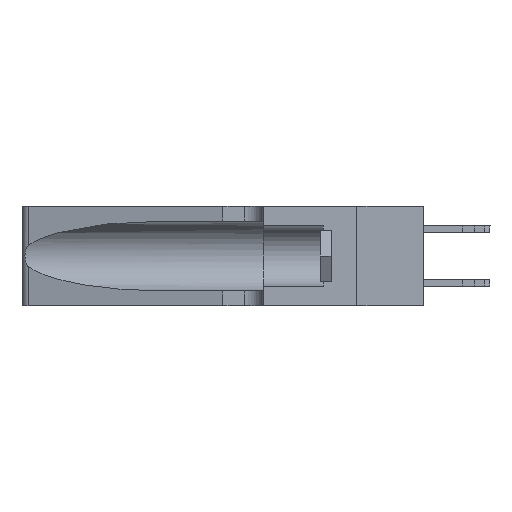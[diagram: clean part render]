
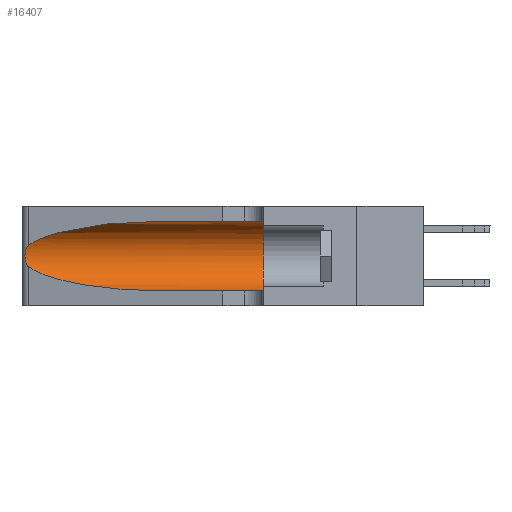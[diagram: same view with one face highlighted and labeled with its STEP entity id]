
A CAD part, left-side view. The second image highlights one B-rep face of the part: STEP entity #16407.
In plain terms, the highlighted cylindrical face has radius 3.308 mm (diameter 6.617 mm), a partial arc.
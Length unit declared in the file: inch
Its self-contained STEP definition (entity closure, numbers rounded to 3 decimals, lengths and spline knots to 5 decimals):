
#221 = CIRCLE ( 'NONE', #20398, 0.13025 ) ;
#550 = CARTESIAN_POINT ( 'NONE',  ( 0.1305, 0.72297, 0.31525 ) ) ;
#918 = VERTEX_POINT ( 'NONE', #16418 ) ;
#952 = EDGE_CURVE ( 'NONE', #918, #15052, #13088, .T. ) ;
#955 = ORIENTED_EDGE ( 'NONE', *, *, #3729, .F. ) ;
#1176 = CYLINDRICAL_SURFACE ( 'NONE', #19075, 0.13025 ) ;
#1247 = CARTESIAN_POINT ( 'NONE',  ( 0.25639, 1.23186, 0.15144 ) ) ;
#1499 = ORIENTED_EDGE ( 'NONE', *, *, #3423, .T. ) ;
#3002 = CARTESIAN_POINT ( 'NONE',  ( 0.26075, 1.23896, 0.178 ) ) ;
#3423 = EDGE_CURVE ( 'NONE', #6405, #12918, #13375, .T. ) ;
#3729 = EDGE_CURVE ( 'NONE', #11415, #15052, #221, .T. ) ;
#3819 = CARTESIAN_POINT ( 'NONE',  ( 0.2373, 1.15595, 0.28018 ) ) ;
#4399 = EDGE_CURVE ( 'NONE', #7703, #11415, #8384, .T. ) ;
#4429 = CARTESIAN_POINT ( 'NONE',  ( 0.25555, 1.22993, 0.14849 ) ) ;
#5075 = DIRECTION ( 'NONE',  ( 0., 0., -1. ) ) ;
#5681 = CARTESIAN_POINT ( 'NONE',  ( 0.25487, 1.22718, 0.14631 ) ) ;
#6241 = CARTESIAN_POINT ( 'NONE',  ( 0.25639, 1.23184, 0.21858 ) ) ;
#6405 = VERTEX_POINT ( 'NONE', #19972 ) ;
#6796 = CARTESIAN_POINT ( 'NONE',  ( 0.18966, 0.96281, 0.31525 ) ) ;
#6901 = CARTESIAN_POINT ( 'NONE',  ( 0.1305, 0.35, 0.31525 ) ) ;
#7072 = ORIENTED_EDGE ( 'NONE', *, *, #15468, .T. ) ;
#7164 =( BOUNDED_CURVE ( )  B_SPLINE_CURVE ( 3, ( #14994, #16622, #8827, #18570 ),
 .UNSPECIFIED., .F., .F. ) 
 B_SPLINE_CURVE_WITH_KNOTS ( ( 4, 4 ),
 ( 3.44316, 4.71239 ),
 .UNSPECIFIED. ) 
 CURVE ( )  GEOMETRIC_REPRESENTATION_ITEM ( )  RATIONAL_B_SPLINE_CURVE ( ( 1., 0.87, 0.87, 1. ) ) 
 REPRESENTATION_ITEM ( '' )  );
#7393 = FACE_OUTER_BOUND ( 'NONE', #14628, .T. ) ;
#7504 = CARTESIAN_POINT ( 'NONE',  ( 0.1305, 1.61858, 0.05475 ) ) ;
#7569 = DIRECTION ( 'NONE',  ( 0., -1., 0. ) ) ;
#7703 = VERTEX_POINT ( 'NONE', #550 ) ;
#7839 = CARTESIAN_POINT ( 'NONE',  ( 0.25854, 1.2359, 0.20912 ) ) ;
#8062 =( BOUNDED_CURVE ( )  B_SPLINE_CURVE ( 3, ( #13434, #6796, #3819, #16614 ),
 .UNSPECIFIED., .F., .T. ) 
 B_SPLINE_CURVE_WITH_KNOTS ( ( 4, 4 ),
 ( 1.5708, 2.84003 ),
 .UNSPECIFIED. ) 
 CURVE ( )  GEOMETRIC_REPRESENTATION_ITEM ( )  RATIONAL_B_SPLINE_CURVE ( ( 1., 0.87, 0.87, 1. ) ) 
 REPRESENTATION_ITEM ( '' )  );
#8350 = DIRECTION ( 'NONE',  ( 0., 1., 0. ) ) ;
#8384 = LINE ( 'NONE', #19009, #18735 ) ;
#8827 = CARTESIAN_POINT ( 'NONE',  ( 0.18966, 0.96281, 0.05475 ) ) ;
#9008 = EDGE_CURVE ( 'NONE', #7703, #6405, #8062, .T. ) ;
#9167 = CARTESIAN_POINT ( 'NONE',  ( 0.25555, 1.22994, 0.2215 ) ) ;
#9451 = CARTESIAN_POINT ( 'NONE',  ( 0.26017, 1.23833, 0.17102 ) ) ;
#9759 = CARTESIAN_POINT ( 'NONE',  ( 0.1305, 1.61858, 0.185 ) ) ;
#9830 = CARTESIAN_POINT ( 'NONE',  ( 0.1305, 0.35, 0.05475 ) ) ;
#10783 = CARTESIAN_POINT ( 'NONE',  ( 0.26018, 1.23835, 0.19895 ) ) ;
#11379 = DIRECTION ( 'NONE',  ( 0., -1., 0. ) ) ;
#11415 = VERTEX_POINT ( 'NONE', #6901 ) ;
#11594 = DIRECTION ( 'NONE',  ( 0., 0., 1. ) ) ;
#12589 = VECTOR ( 'NONE', #7569, 39.37008 ) ;
#12918 = VERTEX_POINT ( 'NONE', #5681 ) ;
#13088 = LINE ( 'NONE', #7504, #12589 ) ;
#13375 = B_SPLINE_CURVE_WITH_KNOTS ( 'NONE', 3,
 ( #15909, #9167, #6241, #17499, #7839, #10783, #19144, #3002, #9451, #20473, #20757, #1247, #4429, #17360 ),
 .UNSPECIFIED., .F., .F.,
 ( 4, 2, 2, 2, 2, 2, 4 ),
 ( 0., 0.00027, 0.00053, 0.00107, 0.0016, 0.00187, 0.00214 ),
 .UNSPECIFIED. ) ;
#13434 = CARTESIAN_POINT ( 'NONE',  ( 0.1305, 0.72297, 0.31525 ) ) ;
#13614 = ORIENTED_EDGE ( 'NONE', *, *, #952, .T. ) ;
#13779 = ORIENTED_EDGE ( 'NONE', *, *, #4399, .F. ) ;
#13998 = DIRECTION ( 'NONE',  ( 0., -1., 0. ) ) ;
#14628 = EDGE_LOOP ( 'NONE', ( #15160, #1499, #7072, #13614, #955, #13779 ) ) ;
#14994 = CARTESIAN_POINT ( 'NONE',  ( 0.25487, 1.22718, 0.14631 ) ) ;
#15052 = VERTEX_POINT ( 'NONE', #9830 ) ;
#15160 = ORIENTED_EDGE ( 'NONE', *, *, #9008, .T. ) ;
#15468 = EDGE_CURVE ( 'NONE', #12918, #918, #7164, .T. ) ;
#15909 = CARTESIAN_POINT ( 'NONE',  ( 0.25487, 1.22718, 0.22369 ) ) ;
#16407 = ADVANCED_FACE ( 'NONE', ( #7393 ), #1176, .F. ) ;
#16418 = CARTESIAN_POINT ( 'NONE',  ( 0.1305, 0.72297, 0.05475 ) ) ;
#16614 = CARTESIAN_POINT ( 'NONE',  ( 0.25487, 1.22718, 0.22369 ) ) ;
#16622 = CARTESIAN_POINT ( 'NONE',  ( 0.2373, 1.15595, 0.08982 ) ) ;
#17360 = CARTESIAN_POINT ( 'NONE',  ( 0.25487, 1.22718, 0.14631 ) ) ;
#17499 = CARTESIAN_POINT ( 'NONE',  ( 0.25787, 1.23484, 0.2124 ) ) ;
#18005 = CARTESIAN_POINT ( 'NONE',  ( 0.1305, 0.35, 0.185 ) ) ;
#18570 = CARTESIAN_POINT ( 'NONE',  ( 0.1305, 0.72297, 0.05475 ) ) ;
#18735 = VECTOR ( 'NONE', #13998, 39.37008 ) ;
#19009 = CARTESIAN_POINT ( 'NONE',  ( 0.1305, 1.61858, 0.31525 ) ) ;
#19075 = AXIS2_PLACEMENT_3D ( 'NONE', #9759, #11379, #5075 ) ;
#19144 = CARTESIAN_POINT ( 'NONE',  ( 0.26075, 1.23896, 0.19203 ) ) ;
#19972 = CARTESIAN_POINT ( 'NONE',  ( 0.25487, 1.22718, 0.22369 ) ) ;
#20398 = AXIS2_PLACEMENT_3D ( 'NONE', #18005, #8350, #11594 ) ;
#20473 = CARTESIAN_POINT ( 'NONE',  ( 0.25856, 1.23593, 0.16098 ) ) ;
#20757 = CARTESIAN_POINT ( 'NONE',  ( 0.25789, 1.23486, 0.15765 ) ) ;
